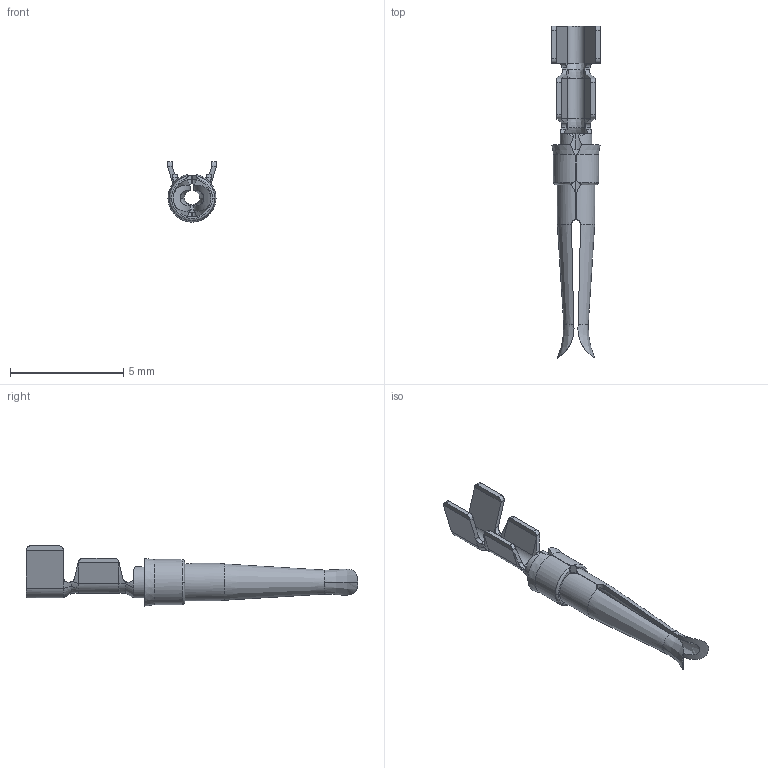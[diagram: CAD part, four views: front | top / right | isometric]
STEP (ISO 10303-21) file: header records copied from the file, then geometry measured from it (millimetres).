
FILE_DESCRIPTION (( 'STEP AP214' ), '1' );
FILE_NAME ('628-292-001.STEP', '2020-09-18T16:00:39', ( '' ), ( '' ), 'SwSTEP 2.0', 'SolidWorks 2020', '' );
FILE_SCHEMA (( 'AUTOMOTIVE_DESIGN' ));
Length unit declared in the file: millimetre
Products named in the file (1): 628-292-001
Bounding box: 2.15 x 14.65 x 2.66 mm (x, y, z)
Volume: 10.9 mm3; surface area: 121.8 mm2
Topology: 1 solids, 1 shells, 159 faces, 421 edges, 264 vertices
Faces by surface type: plane 54, bspline 52, cylinder 47, cone 6
Entity records: 6479 total; most frequent: CARTESIAN_POINT 2849, ORIENTED_EDGE 842, DIRECTION 488, EDGE_CURVE 421, VERTEX_POINT 264, B_SPLINE_CURVE_WITH_KNOTS 186, VECTOR 178, LINE 178
